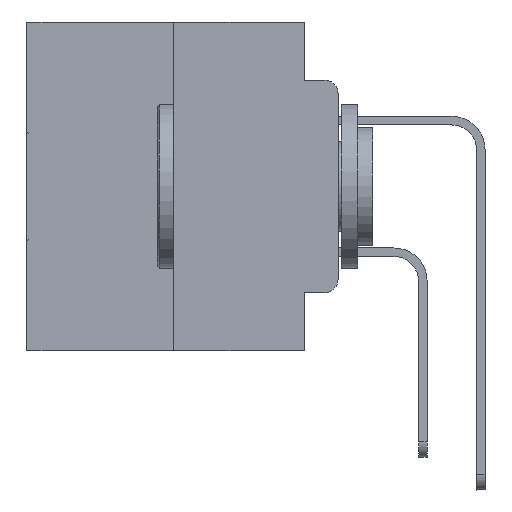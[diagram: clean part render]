
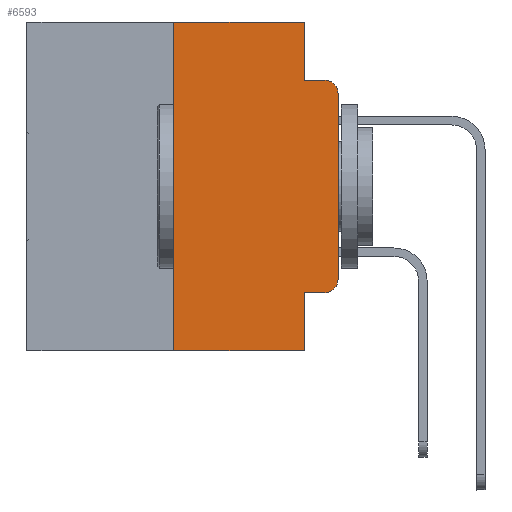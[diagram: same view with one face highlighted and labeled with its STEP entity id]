
A CAD part, left-side view. The second image highlights one B-rep face of the part: STEP entity #6593.
In plain terms, the highlighted planar face has unit normal (-1, 0, 0).
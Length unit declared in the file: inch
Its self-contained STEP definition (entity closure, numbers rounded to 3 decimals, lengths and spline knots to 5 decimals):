
#162 = ORIENTED_EDGE ( 'NONE', *, *, #12099, .T. ) ;
#996 = ORIENTED_EDGE ( 'NONE', *, *, #7096, .T. ) ;
#998 = CARTESIAN_POINT ( 'NONE',  ( 0., 0.051, 0. ) ) ;
#1522 = CARTESIAN_POINT ( 'NONE',  ( 0., 0.25, 0. ) ) ;
#1567 = VECTOR ( 'NONE', #24438, 39.37008 ) ;
#3144 = CARTESIAN_POINT ( 'NONE',  ( 0., 0.051, 0. ) ) ;
#3285 = CARTESIAN_POINT ( 'NONE',  ( 0., 0.25, -0.5 ) ) ;
#3534 = DIRECTION ( 'NONE',  ( 0., -1., 0. ) ) ;
#3973 = VERTEX_POINT ( 'NONE', #8512 ) ;
#4060 = CARTESIAN_POINT ( 'NONE',  ( 0., 0.02, -0.1085 ) ) ;
#4592 = AXIS2_PLACEMENT_3D ( 'NONE', #16395, #6421, #23951 ) ;
#4808 = DIRECTION ( 'NONE',  ( 0., -1., 0. ) ) ;
#4881 = VERTEX_POINT ( 'NONE', #22134 ) ;
#5437 = ORIENTED_EDGE ( 'NONE', *, *, #15935, .T. ) ;
#5561 = FACE_OUTER_BOUND ( 'NONE', #21237, .T. ) ;
#5629 = DIRECTION ( 'NONE',  ( 0., -1., 0. ) ) ;
#5855 = CARTESIAN_POINT ( 'NONE',  ( 0., 0.02, -0.3915 ) ) ;
#6328 = CARTESIAN_POINT ( 'NONE',  ( 0., 0.051, 0. ) ) ;
#6421 = DIRECTION ( 'NONE',  ( 1., 0., 0. ) ) ;
#6593 = ADVANCED_FACE ( 'NONE', ( #5561 ), #21423, .F. ) ;
#6639 = DIRECTION ( 'NONE',  ( 0., 0., -1. ) ) ;
#7096 = EDGE_CURVE ( 'NONE', #27805, #4881, #30241, .T. ) ;
#7672 = VECTOR ( 'NONE', #18665, 39.37008 ) ;
#7742 = LINE ( 'NONE', #9784, #26978 ) ;
#8364 = DIRECTION ( 'NONE',  ( 0., 0., -1. ) ) ;
#8385 = CARTESIAN_POINT ( 'NONE',  ( 0., 0., 0. ) ) ;
#8512 = CARTESIAN_POINT ( 'NONE',  ( 0., 0., -0.1085 ) ) ;
#8943 = ORIENTED_EDGE ( 'NONE', *, *, #23901, .T. ) ;
#9120 = LINE ( 'NONE', #16887, #1567 ) ;
#9714 = ORIENTED_EDGE ( 'NONE', *, *, #22188, .F. ) ;
#9784 = CARTESIAN_POINT ( 'NONE',  ( 0., 0.051, -0.4115 ) ) ;
#10507 = ORIENTED_EDGE ( 'NONE', *, *, #21739, .F. ) ;
#10887 = DIRECTION ( 'NONE',  ( 0., 0., 1. ) ) ;
#12099 = EDGE_CURVE ( 'NONE', #25298, #27805, #7742, .T. ) ;
#12260 = VECTOR ( 'NONE', #5629, 39.37008 ) ;
#12851 = ORIENTED_EDGE ( 'NONE', *, *, #13776, .F. ) ;
#13250 = VERTEX_POINT ( 'NONE', #1522 ) ;
#13776 = EDGE_CURVE ( 'NONE', #25298, #28837, #31915, .T. ) ;
#14521 = VECTOR ( 'NONE', #10887, 39.37008 ) ;
#15266 = CIRCLE ( 'NONE', #28648, 0.02 ) ;
#15481 = EDGE_CURVE ( 'NONE', #28976, #13250, #9120, .T. ) ;
#15935 = EDGE_CURVE ( 'NONE', #28976, #28837, #21642, .T. ) ;
#16395 = CARTESIAN_POINT ( 'NONE',  ( 0., 0.473, 0. ) ) ;
#16887 = CARTESIAN_POINT ( 'NONE',  ( 0., 0.25, 0. ) ) ;
#17342 = CARTESIAN_POINT ( 'NONE',  ( 0., 0.051, -0.0885 ) ) ;
#17381 = VECTOR ( 'NONE', #4808, 39.37008 ) ;
#18112 = CARTESIAN_POINT ( 'NONE',  ( 0., 0.02, -0.4115 ) ) ;
#18162 = LINE ( 'NONE', #17342, #17381 ) ;
#18665 = DIRECTION ( 'NONE',  ( 0., 0., -1. ) ) ;
#18668 = VECTOR ( 'NONE', #18813, 39.37008 ) ;
#18813 = DIRECTION ( 'NONE',  ( 0., 0., -1. ) ) ;
#20229 = CARTESIAN_POINT ( 'NONE',  ( 0., 0.02, -0.0885 ) ) ;
#20538 = EDGE_CURVE ( 'NONE', #24327, #24145, #26909, .T. ) ;
#21024 = CARTESIAN_POINT ( 'NONE',  ( 0., 0.473, -0.5 ) ) ;
#21222 = LINE ( 'NONE', #8385, #14521 ) ;
#21237 = EDGE_LOOP ( 'NONE', ( #28161, #8943, #9714, #23061, #10507, #24656, #5437, #12851, #162, #996 ) ) ;
#21423 = PLANE ( 'NONE',  #4592 ) ;
#21628 = DIRECTION ( 'NONE',  ( -1., 0., 0. ) ) ;
#21642 = LINE ( 'NONE', #21024, #27537 ) ;
#21739 = EDGE_CURVE ( 'NONE', #13250, #24327, #24845, .T. ) ;
#22134 = CARTESIAN_POINT ( 'NONE',  ( 0., 0., -0.3915 ) ) ;
#22188 = EDGE_CURVE ( 'NONE', #24145, #22951, #18162, .T. ) ;
#22448 = AXIS2_PLACEMENT_3D ( 'NONE', #5855, #23366, #8364 ) ;
#22843 = CARTESIAN_POINT ( 'NONE',  ( 0., 0.051, -0.5 ) ) ;
#22951 = VERTEX_POINT ( 'NONE', #20229 ) ;
#23061 = ORIENTED_EDGE ( 'NONE', *, *, #20538, .F. ) ;
#23140 = CARTESIAN_POINT ( 'NONE',  ( 0., 0.473, 0. ) ) ;
#23366 = DIRECTION ( 'NONE',  ( -1., 0., 0. ) ) ;
#23901 = EDGE_CURVE ( 'NONE', #3973, #22951, #15266, .T. ) ;
#23951 = DIRECTION ( 'NONE',  ( 0., 0., -1. ) ) ;
#24145 = VERTEX_POINT ( 'NONE', #25122 ) ;
#24327 = VERTEX_POINT ( 'NONE', #3144 ) ;
#24438 = DIRECTION ( 'NONE',  ( 0., 0., 1. ) ) ;
#24656 = ORIENTED_EDGE ( 'NONE', *, *, #15481, .F. ) ;
#24832 = DIRECTION ( 'NONE',  ( 0., -1., 0. ) ) ;
#24845 = LINE ( 'NONE', #23140, #12260 ) ;
#25122 = CARTESIAN_POINT ( 'NONE',  ( 0., 0.051, -0.0885 ) ) ;
#25298 = VERTEX_POINT ( 'NONE', #31789 ) ;
#26909 = LINE ( 'NONE', #998, #7672 ) ;
#26978 = VECTOR ( 'NONE', #24832, 39.37008 ) ;
#27263 = EDGE_CURVE ( 'NONE', #4881, #3973, #21222, .T. ) ;
#27537 = VECTOR ( 'NONE', #3534, 39.37008 ) ;
#27805 = VERTEX_POINT ( 'NONE', #18112 ) ;
#28161 = ORIENTED_EDGE ( 'NONE', *, *, #27263, .T. ) ;
#28648 = AXIS2_PLACEMENT_3D ( 'NONE', #4060, #21628, #6639 ) ;
#28837 = VERTEX_POINT ( 'NONE', #22843 ) ;
#28976 = VERTEX_POINT ( 'NONE', #3285 ) ;
#30241 = CIRCLE ( 'NONE', #22448, 0.02 ) ;
#31789 = CARTESIAN_POINT ( 'NONE',  ( 0., 0.051, -0.4115 ) ) ;
#31915 = LINE ( 'NONE', #6328, #18668 ) ;
